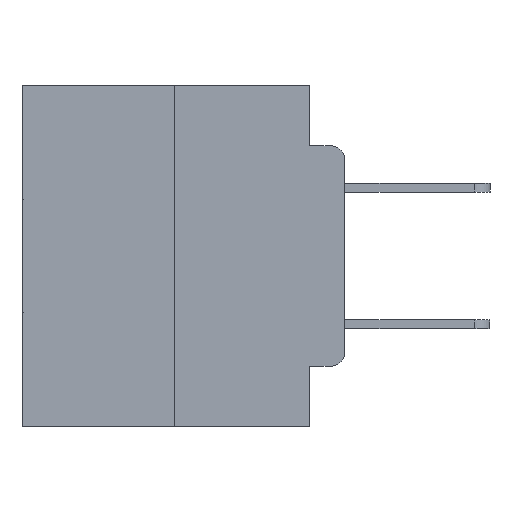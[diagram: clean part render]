
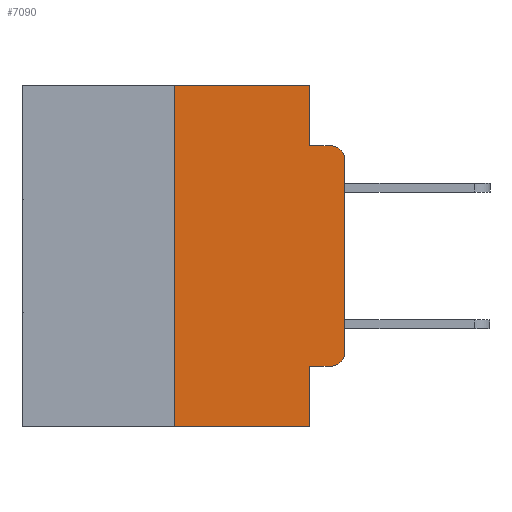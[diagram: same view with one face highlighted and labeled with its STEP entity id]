
A CAD part, left-side view. The second image highlights one B-rep face of the part: STEP entity #7090.
In plain terms, the highlighted planar face has unit normal (-1, 0, 0).
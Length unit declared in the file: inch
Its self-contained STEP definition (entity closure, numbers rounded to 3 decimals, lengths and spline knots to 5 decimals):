
#127 = DIRECTION ( 'NONE',  ( 0., 0., 1. ) ) ;
#217 = CARTESIAN_POINT ( 'NONE',  ( 0., 0.473, 0. ) ) ;
#386 = CARTESIAN_POINT ( 'NONE',  ( 0., 0.051, 0. ) ) ;
#601 = VECTOR ( 'NONE', #14010, 39.37008 ) ;
#853 = VECTOR ( 'NONE', #5855, 39.37008 ) ;
#1343 = VERTEX_POINT ( 'NONE', #8425 ) ;
#1374 = AXIS2_PLACEMENT_3D ( 'NONE', #217, #11387, #26386 ) ;
#1793 = ORIENTED_EDGE ( 'NONE', *, *, #14500, .F. ) ;
#1815 = AXIS2_PLACEMENT_3D ( 'NONE', #9467, #24576, #11696 ) ;
#1821 = VERTEX_POINT ( 'NONE', #6038 ) ;
#2020 = CIRCLE ( 'NONE', #18307, 0.02 ) ;
#2033 = LINE ( 'NONE', #11755, #601 ) ;
#2981 = VECTOR ( 'NONE', #9341, 39.37008 ) ;
#3139 = CARTESIAN_POINT ( 'NONE',  ( 0., 0.02, -0.4115 ) ) ;
#3471 = CARTESIAN_POINT ( 'NONE',  ( 0., 0.02, -0.1085 ) ) ;
#4410 = VECTOR ( 'NONE', #8317, 39.37008 ) ;
#4589 = ORIENTED_EDGE ( 'NONE', *, *, #18856, .F. ) ;
#5097 = LINE ( 'NONE', #5984, #4410 ) ;
#5242 = CARTESIAN_POINT ( 'NONE',  ( 0., 0.25, 0. ) ) ;
#5670 = EDGE_CURVE ( 'NONE', #23021, #27047, #12791, .T. ) ;
#5675 = DIRECTION ( 'NONE',  ( 0., 0., -1. ) ) ;
#5767 = CARTESIAN_POINT ( 'NONE',  ( 0., 0.051, -0.0885 ) ) ;
#5855 = DIRECTION ( 'NONE',  ( 0., -1., 0. ) ) ;
#5897 = DIRECTION ( 'NONE',  ( 0., -1., 0. ) ) ;
#5984 = CARTESIAN_POINT ( 'NONE',  ( 0., 0.473, 0. ) ) ;
#6038 = CARTESIAN_POINT ( 'NONE',  ( 0., 0.25, -0.5 ) ) ;
#6291 = ORIENTED_EDGE ( 'NONE', *, *, #8670, .T. ) ;
#6651 = CIRCLE ( 'NONE', #1815, 0.02 ) ;
#6777 = LINE ( 'NONE', #14585, #853 ) ;
#7090 = ADVANCED_FACE ( 'NONE', ( #11338 ), #24273, .F. ) ;
#7138 = VERTEX_POINT ( 'NONE', #17718 ) ;
#7350 = ORIENTED_EDGE ( 'NONE', *, *, #15945, .F. ) ;
#8317 = DIRECTION ( 'NONE',  ( 0., -1., 0. ) ) ;
#8425 = CARTESIAN_POINT ( 'NONE',  ( 0., 0.02, -0.0885 ) ) ;
#8670 = EDGE_CURVE ( 'NONE', #27047, #1343, #2020, .T. ) ;
#8783 = CARTESIAN_POINT ( 'NONE',  ( 0., 0.25, 0. ) ) ;
#9341 = DIRECTION ( 'NONE',  ( 0., 0., -1. ) ) ;
#9415 = VECTOR ( 'NONE', #19275, 39.37008 ) ;
#9467 = CARTESIAN_POINT ( 'NONE',  ( 0., 0.02, -0.3915 ) ) ;
#10046 = CARTESIAN_POINT ( 'NONE',  ( 0., 0., -0.1085 ) ) ;
#10062 = VECTOR ( 'NONE', #5897, 39.37008 ) ;
#10095 = LINE ( 'NONE', #23487, #9415 ) ;
#10135 = EDGE_LOOP ( 'NONE', ( #16537, #6291, #1793, #24929, #21286, #4589, #16898, #7350, #25266, #14538 ) ) ;
#11338 = FACE_OUTER_BOUND ( 'NONE', #10135, .T. ) ;
#11387 = DIRECTION ( 'NONE',  ( 1., 0., 0. ) ) ;
#11696 = DIRECTION ( 'NONE',  ( 0., 0., -1. ) ) ;
#11755 = CARTESIAN_POINT ( 'NONE',  ( 0., 0.051, -0.0885 ) ) ;
#11831 = VECTOR ( 'NONE', #26019, 39.37008 ) ;
#12791 = LINE ( 'NONE', #24112, #23540 ) ;
#13081 = EDGE_CURVE ( 'NONE', #20308, #14061, #10095, .T. ) ;
#14010 = DIRECTION ( 'NONE',  ( 0., -1., 0. ) ) ;
#14061 = VERTEX_POINT ( 'NONE', #5767 ) ;
#14500 = EDGE_CURVE ( 'NONE', #14061, #1343, #2033, .T. ) ;
#14538 = ORIENTED_EDGE ( 'NONE', *, *, #20293, .T. ) ;
#14585 = CARTESIAN_POINT ( 'NONE',  ( 0., 0.473, -0.5 ) ) ;
#15929 = CARTESIAN_POINT ( 'NONE',  ( 0., 0.051, 0. ) ) ;
#15945 = EDGE_CURVE ( 'NONE', #27170, #7138, #25389, .T. ) ;
#16537 = ORIENTED_EDGE ( 'NONE', *, *, #5670, .T. ) ;
#16710 = VERTEX_POINT ( 'NONE', #5242 ) ;
#16898 = ORIENTED_EDGE ( 'NONE', *, *, #24741, .T. ) ;
#17718 = CARTESIAN_POINT ( 'NONE',  ( 0., 0.051, -0.5 ) ) ;
#18261 = LINE ( 'NONE', #8783, #11831 ) ;
#18307 = AXIS2_PLACEMENT_3D ( 'NONE', #3471, #18771, #5675 ) ;
#18771 = DIRECTION ( 'NONE',  ( -1., 0., 0. ) ) ;
#18856 = EDGE_CURVE ( 'NONE', #1821, #16710, #18261, .T. ) ;
#19275 = DIRECTION ( 'NONE',  ( 0., 0., -1. ) ) ;
#20293 = EDGE_CURVE ( 'NONE', #20929, #23021, #6651, .T. ) ;
#20308 = VERTEX_POINT ( 'NONE', #15929 ) ;
#20929 = VERTEX_POINT ( 'NONE', #3139 ) ;
#21286 = ORIENTED_EDGE ( 'NONE', *, *, #24190, .F. ) ;
#21751 = EDGE_CURVE ( 'NONE', #27170, #20929, #27842, .T. ) ;
#23021 = VERTEX_POINT ( 'NONE', #26682 ) ;
#23487 = CARTESIAN_POINT ( 'NONE',  ( 0., 0.051, 0. ) ) ;
#23540 = VECTOR ( 'NONE', #127, 39.37008 ) ;
#24112 = CARTESIAN_POINT ( 'NONE',  ( 0., 0., 0. ) ) ;
#24190 = EDGE_CURVE ( 'NONE', #16710, #20308, #5097, .T. ) ;
#24273 = PLANE ( 'NONE',  #1374 ) ;
#24576 = DIRECTION ( 'NONE',  ( -1., 0., 0. ) ) ;
#24741 = EDGE_CURVE ( 'NONE', #1821, #7138, #6777, .T. ) ;
#24929 = ORIENTED_EDGE ( 'NONE', *, *, #13081, .F. ) ;
#25266 = ORIENTED_EDGE ( 'NONE', *, *, #21751, .T. ) ;
#25389 = LINE ( 'NONE', #386, #2981 ) ;
#25484 = CARTESIAN_POINT ( 'NONE',  ( 0., 0.051, -0.4115 ) ) ;
#26019 = DIRECTION ( 'NONE',  ( 0., 0., 1. ) ) ;
#26386 = DIRECTION ( 'NONE',  ( 0., 0., -1. ) ) ;
#26682 = CARTESIAN_POINT ( 'NONE',  ( 0., 0., -0.3915 ) ) ;
#27047 = VERTEX_POINT ( 'NONE', #10046 ) ;
#27170 = VERTEX_POINT ( 'NONE', #25484 ) ;
#27409 = CARTESIAN_POINT ( 'NONE',  ( 0., 0.051, -0.4115 ) ) ;
#27842 = LINE ( 'NONE', #27409, #10062 ) ;
